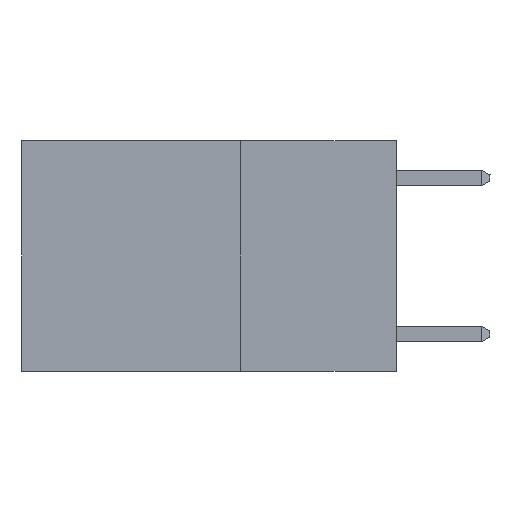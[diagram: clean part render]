
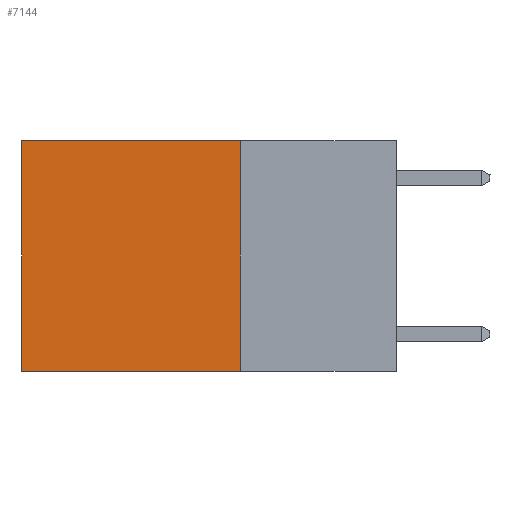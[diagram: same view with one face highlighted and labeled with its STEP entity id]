
A CAD part, left-side view. The second image highlights one B-rep face of the part: STEP entity #7144.
In plain terms, the highlighted planar face has unit normal (-1, 0, 0).
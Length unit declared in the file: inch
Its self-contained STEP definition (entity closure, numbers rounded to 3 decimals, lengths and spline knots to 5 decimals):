
#292 = DIRECTION ( 'NONE',  ( 0., 1., 0. ) ) ;
#483 = VECTOR ( 'NONE', #3697, 39.37008 ) ;
#556 = DIRECTION ( 'NONE',  ( 0., 0., -1. ) ) ;
#644 = CARTESIAN_POINT ( 'NONE',  ( 0.2625, 0.6, 0. ) ) ;
#675 = DIRECTION ( 'NONE',  ( 0., 0., -1. ) ) ;
#1750 = EDGE_CURVE ( 'NONE', #11512, #5409, #4997, .T. ) ;
#1910 = ORIENTED_EDGE ( 'NONE', *, *, #9441, .F. ) ;
#2646 = VERTEX_POINT ( 'NONE', #6626 ) ;
#3015 = ORIENTED_EDGE ( 'NONE', *, *, #1750, .F. ) ;
#3405 = CARTESIAN_POINT ( 'NONE',  ( 0.2625, 0.25, -0.37 ) ) ;
#3695 = DIRECTION ( 'NONE',  ( 0., 0., -1. ) ) ;
#3697 = DIRECTION ( 'NONE',  ( 0., 1., 0. ) ) ;
#3882 = VERTEX_POINT ( 'NONE', #644 ) ;
#4362 = EDGE_CURVE ( 'NONE', #11512, #3882, #8517, .T. ) ;
#4997 = LINE ( 'NONE', #10028, #9804 ) ;
#5409 = VERTEX_POINT ( 'NONE', #3405 ) ;
#5502 = ORIENTED_EDGE ( 'NONE', *, *, #9783, .T. ) ;
#5602 = CARTESIAN_POINT ( 'NONE',  ( 0.2625, 0.25, 0. ) ) ;
#5805 = EDGE_LOOP ( 'NONE', ( #5502, #1910, #3015, #10365 ) ) ;
#6107 = CARTESIAN_POINT ( 'NONE',  ( 0.2625, 0.25, -0.37 ) ) ;
#6365 = DIRECTION ( 'NONE',  ( 1., 0., 0. ) ) ;
#6626 = CARTESIAN_POINT ( 'NONE',  ( 0.2625, 0.6, -0.37 ) ) ;
#6820 = FACE_OUTER_BOUND ( 'NONE', #5805, .T. ) ;
#7144 = ADVANCED_FACE ( 'NONE', ( #6820 ), #12082, .F. ) ;
#8517 = LINE ( 'NONE', #5602, #483 ) ;
#9225 = CARTESIAN_POINT ( 'NONE',  ( 0.2625, 0.25, 0. ) ) ;
#9441 = EDGE_CURVE ( 'NONE', #5409, #2646, #10341, .T. ) ;
#9744 = AXIS2_PLACEMENT_3D ( 'NONE', #9225, #6365, #556 ) ;
#9783 = EDGE_CURVE ( 'NONE', #3882, #2646, #11813, .T. ) ;
#9804 = VECTOR ( 'NONE', #675, 39.37008 ) ;
#9805 = CARTESIAN_POINT ( 'NONE',  ( 0.2625, 0.25, 0. ) ) ;
#10028 = CARTESIAN_POINT ( 'NONE',  ( 0.2625, 0.25, 0. ) ) ;
#10031 = VECTOR ( 'NONE', #292, 39.37008 ) ;
#10341 = LINE ( 'NONE', #6107, #10031 ) ;
#10365 = ORIENTED_EDGE ( 'NONE', *, *, #4362, .T. ) ;
#10408 = CARTESIAN_POINT ( 'NONE',  ( 0.2625, 0.6, 0. ) ) ;
#11512 = VERTEX_POINT ( 'NONE', #9805 ) ;
#11523 = VECTOR ( 'NONE', #3695, 39.37008 ) ;
#11813 = LINE ( 'NONE', #10408, #11523 ) ;
#12082 = PLANE ( 'NONE',  #9744 ) ;
